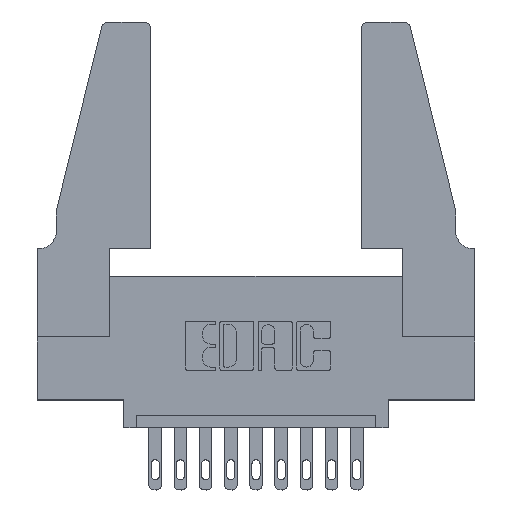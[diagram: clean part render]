
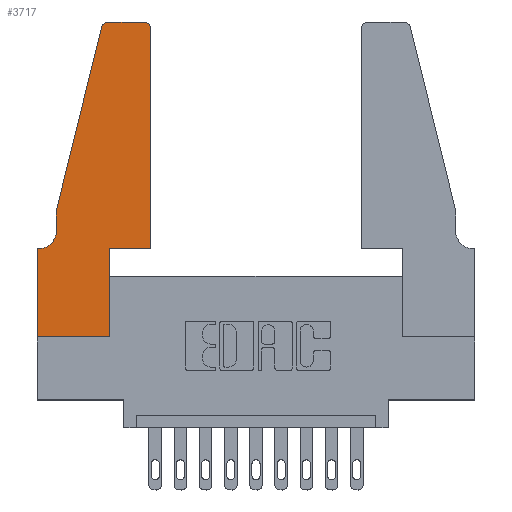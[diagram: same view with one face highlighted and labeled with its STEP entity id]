
A CAD part, top view. The second image highlights one B-rep face of the part: STEP entity #3717.
In plain terms, the highlighted planar face has unit normal (0, 0, 1).
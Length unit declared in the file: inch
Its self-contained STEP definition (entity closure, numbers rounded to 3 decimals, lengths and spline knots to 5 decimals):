
#371 = CARTESIAN_POINT ( 'NONE',  ( 0.4505, 0.35, 0.37 ) ) ;
#398 = DIRECTION ( 'NONE',  ( 0., -1., 0. ) ) ;
#654 = ORIENTED_EDGE ( 'NONE', *, *, #12667, .T. ) ;
#805 = ORIENTED_EDGE ( 'NONE', *, *, #6566, .T. ) ;
#885 = CARTESIAN_POINT ( 'NONE',  ( 0.4205, 1.22, 0.37 ) ) ;
#968 = VERTEX_POINT ( 'NONE', #11176 ) ;
#996 = AXIS2_PLACEMENT_3D ( 'NONE', #885, #2911, #4018 ) ;
#1023 = DIRECTION ( 'NONE',  ( -0.239, -0.971, 0. ) ) ;
#1108 = VECTOR ( 'NONE', #8968, 39.37008 ) ;
#1172 = CARTESIAN_POINT ( 'NONE',  ( 0.0755, 0.5, 0.37 ) ) ;
#1540 = CARTESIAN_POINT ( 'NONE',  ( 0.0755, 0.5, 0.37 ) ) ;
#1821 = DIRECTION ( 'NONE',  ( -1., 0., 0. ) ) ;
#1863 = ORIENTED_EDGE ( 'NONE', *, *, #7676, .T. ) ;
#1959 = EDGE_CURVE ( 'NONE', #968, #5667, #2778, .T. ) ;
#2427 = ORIENTED_EDGE ( 'NONE', *, *, #1959, .T. ) ;
#2430 = EDGE_CURVE ( 'NONE', #9907, #968, #8509, .T. ) ;
#2470 = LINE ( 'NONE', #7142, #4242 ) ;
#2483 = LINE ( 'NONE', #4863, #11226 ) ;
#2759 = LINE ( 'NONE', #10049, #7269 ) ;
#2778 = LINE ( 'NONE', #10339, #7905 ) ;
#2881 = CARTESIAN_POINT ( 'NONE',  ( 0.2865, 0., 0.37 ) ) ;
#2911 = DIRECTION ( 'NONE',  ( 0., 0., 1. ) ) ;
#2959 = DIRECTION ( 'NONE',  ( 0., -1., 0. ) ) ;
#3650 = AXIS2_PLACEMENT_3D ( 'NONE', #11339, #9127, #10314 ) ;
#3717 = ADVANCED_FACE ( 'NONE', ( #4623 ), #8976, .T. ) ;
#3731 = CARTESIAN_POINT ( 'NONE',  ( 0.284, 1.25, 0.37 ) ) ;
#3858 = DIRECTION ( 'NONE',  ( 1., 0., 0. ) ) ;
#3868 = LINE ( 'NONE', #1540, #6955 ) ;
#3871 = VERTEX_POINT ( 'NONE', #10341 ) ;
#3955 = VERTEX_POINT ( 'NONE', #1172 ) ;
#3973 = CARTESIAN_POINT ( 'NONE',  ( 0.4505, 1.22, 0.37 ) ) ;
#3993 = DIRECTION ( 'NONE',  ( 0., 0., 1. ) ) ;
#4008 = VERTEX_POINT ( 'NONE', #7543 ) ;
#4018 = DIRECTION ( 'NONE',  ( 1., 0., 0. ) ) ;
#4203 = ORIENTED_EDGE ( 'NONE', *, *, #13143, .T. ) ;
#4242 = VECTOR ( 'NONE', #1023, 39.37008 ) ;
#4334 = VERTEX_POINT ( 'NONE', #6267 ) ;
#4623 = FACE_OUTER_BOUND ( 'NONE', #6626, .T. ) ;
#4731 = CARTESIAN_POINT ( 'NONE',  ( 0.25487, 1.22718, 0.37 ) ) ;
#4863 = CARTESIAN_POINT ( 'NONE',  ( 0.4505, 0.35, 0.37 ) ) ;
#4871 = DIRECTION ( 'NONE',  ( 0., 1., 0. ) ) ;
#4912 = CARTESIAN_POINT ( 'NONE',  ( 0., 0.35, 0.37 ) ) ;
#4929 = CARTESIAN_POINT ( 'NONE',  ( 0.2865, 0.35, 0.37 ) ) ;
#4948 = DIRECTION ( 'NONE',  ( -1., 0., 0. ) ) ;
#5279 = VERTEX_POINT ( 'NONE', #3973 ) ;
#5447 = VERTEX_POINT ( 'NONE', #4731 ) ;
#5593 = CARTESIAN_POINT ( 'NONE',  ( 0.0755, 0.35, 0.37 ) ) ;
#5667 = VERTEX_POINT ( 'NONE', #2881 ) ;
#5686 = EDGE_CURVE ( 'NONE', #4008, #6598, #2483, .T. ) ;
#5758 = DIRECTION ( 'NONE',  ( -1., 0., 0. ) ) ;
#6081 = EDGE_CURVE ( 'NONE', #5447, #3955, #2470, .T. ) ;
#6267 = CARTESIAN_POINT ( 'NONE',  ( 0.0755, 0.42, 0.37 ) ) ;
#6476 = AXIS2_PLACEMENT_3D ( 'NONE', #4912, #3993, #13289 ) ;
#6566 = EDGE_CURVE ( 'NONE', #11935, #5447, #7148, .T. ) ;
#6598 = VERTEX_POINT ( 'NONE', #371 ) ;
#6626 = EDGE_LOOP ( 'NONE', ( #7435, #805, #13009, #7373, #1863, #654, #8823, #2427, #4203, #7235, #8962, #10157 ) ) ;
#6823 = DIRECTION ( 'NONE',  ( 0., 0., -1. ) ) ;
#6955 = VECTOR ( 'NONE', #398, 39.37008 ) ;
#7136 = LINE ( 'NONE', #5593, #10652 ) ;
#7142 = CARTESIAN_POINT ( 'NONE',  ( 0.0755, 0.5, 0.37 ) ) ;
#7148 = CIRCLE ( 'NONE', #3650, 0.03 ) ;
#7193 = EDGE_CURVE ( 'NONE', #3871, #11935, #11338, .T. ) ;
#7235 = ORIENTED_EDGE ( 'NONE', *, *, #5686, .T. ) ;
#7269 = VECTOR ( 'NONE', #4871, 39.37008 ) ;
#7373 = ORIENTED_EDGE ( 'NONE', *, *, #7598, .T. ) ;
#7435 = ORIENTED_EDGE ( 'NONE', *, *, #7193, .T. ) ;
#7543 = CARTESIAN_POINT ( 'NONE',  ( 0.2865, 0.35, 0.37 ) ) ;
#7598 = EDGE_CURVE ( 'NONE', #3955, #4334, #3868, .T. ) ;
#7676 = EDGE_CURVE ( 'NONE', #4334, #7898, #8859, .T. ) ;
#7873 = CARTESIAN_POINT ( 'NONE',  ( 0.0055, 0.35, 0.37 ) ) ;
#7898 = VERTEX_POINT ( 'NONE', #7873 ) ;
#7905 = VECTOR ( 'NONE', #11323, 39.37008 ) ;
#8075 = CARTESIAN_POINT ( 'NONE',  ( 0., 0., 0.37 ) ) ;
#8509 = LINE ( 'NONE', #8075, #10977 ) ;
#8535 = VECTOR ( 'NONE', #4948, 39.37008 ) ;
#8747 = AXIS2_PLACEMENT_3D ( 'NONE', #12135, #6823, #1821 ) ;
#8823 = ORIENTED_EDGE ( 'NONE', *, *, #2430, .T. ) ;
#8859 = CIRCLE ( 'NONE', #8747, 0.07 ) ;
#8962 = ORIENTED_EDGE ( 'NONE', *, *, #12419, .T. ) ;
#8968 = DIRECTION ( 'NONE',  ( 0., 1., 0. ) ) ;
#8976 = PLANE ( 'NONE',  #6476 ) ;
#9003 = LINE ( 'NONE', #4929, #1108 ) ;
#9127 = DIRECTION ( 'NONE',  ( 0., 0., 1. ) ) ;
#9506 = EDGE_CURVE ( 'NONE', #5279, #3871, #12375, .T. ) ;
#9907 = VERTEX_POINT ( 'NONE', #10603 ) ;
#10049 = CARTESIAN_POINT ( 'NONE',  ( 0.4505, 0.35, 0.37 ) ) ;
#10081 = CARTESIAN_POINT ( 'NONE',  ( 0.2605, 1.25, 0.37 ) ) ;
#10157 = ORIENTED_EDGE ( 'NONE', *, *, #9506, .T. ) ;
#10314 = DIRECTION ( 'NONE',  ( 1., 0., 0. ) ) ;
#10339 = CARTESIAN_POINT ( 'NONE',  ( 0., 0., 0.37 ) ) ;
#10341 = CARTESIAN_POINT ( 'NONE',  ( 0.4205, 1.25, 0.37 ) ) ;
#10603 = CARTESIAN_POINT ( 'NONE',  ( 0., 0.35, 0.37 ) ) ;
#10652 = VECTOR ( 'NONE', #5758, 39.37008 ) ;
#10977 = VECTOR ( 'NONE', #2959, 39.37008 ) ;
#11176 = CARTESIAN_POINT ( 'NONE',  ( 0., 0., 0.37 ) ) ;
#11226 = VECTOR ( 'NONE', #3858, 39.37008 ) ;
#11323 = DIRECTION ( 'NONE',  ( 1., 0., 0. ) ) ;
#11338 = LINE ( 'NONE', #10081, #8535 ) ;
#11339 = CARTESIAN_POINT ( 'NONE',  ( 0.284, 1.22, 0.37 ) ) ;
#11935 = VERTEX_POINT ( 'NONE', #3731 ) ;
#12135 = CARTESIAN_POINT ( 'NONE',  ( 0.0055, 0.42, 0.37 ) ) ;
#12375 = CIRCLE ( 'NONE', #996, 0.03 ) ;
#12419 = EDGE_CURVE ( 'NONE', #6598, #5279, #2759, .T. ) ;
#12667 = EDGE_CURVE ( 'NONE', #7898, #9907, #7136, .T. ) ;
#13009 = ORIENTED_EDGE ( 'NONE', *, *, #6081, .T. ) ;
#13143 = EDGE_CURVE ( 'NONE', #5667, #4008, #9003, .T. ) ;
#13289 = DIRECTION ( 'NONE',  ( 1., 0., 0. ) ) ;
